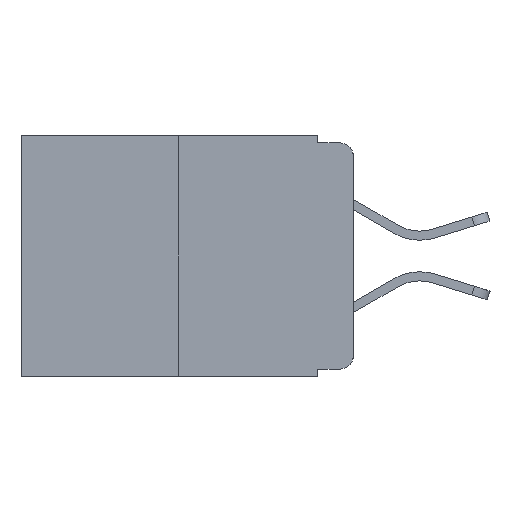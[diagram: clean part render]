
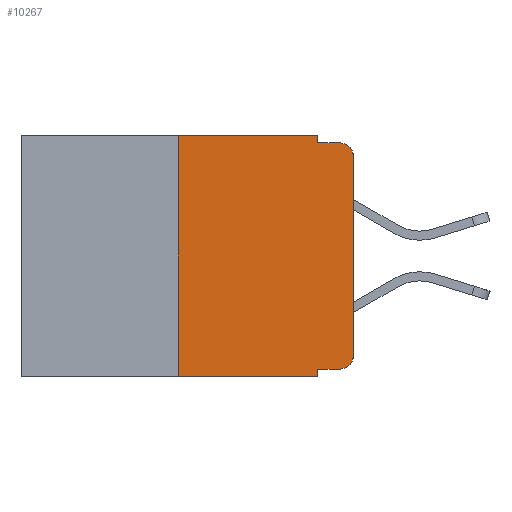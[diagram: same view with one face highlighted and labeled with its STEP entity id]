
A CAD part, left-side view. The second image highlights one B-rep face of the part: STEP entity #10267.
In plain terms, the highlighted planar face has unit normal (-1, 0, 0).
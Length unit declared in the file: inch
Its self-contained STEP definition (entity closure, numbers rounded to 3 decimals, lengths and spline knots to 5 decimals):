
#86 = CARTESIAN_POINT ( 'NONE',  ( 0., 0.051, -0.343 ) ) ;
#326 = CARTESIAN_POINT ( 'NONE',  ( 0., 0.02, -0.333 ) ) ;
#741 = CARTESIAN_POINT ( 'NONE',  ( 0., 0.02, -0.01 ) ) ;
#762 = DIRECTION ( 'NONE',  ( 0., 0., -1. ) ) ;
#869 = VERTEX_POINT ( 'NONE', #6838 ) ;
#930 = LINE ( 'NONE', #11428, #10359 ) ;
#1096 = DIRECTION ( 'NONE',  ( 0., -1., 0. ) ) ;
#1146 = DIRECTION ( 'NONE',  ( 0., 0., -1. ) ) ;
#1485 = EDGE_CURVE ( 'NONE', #869, #4838, #7308, .T. ) ;
#1521 = DIRECTION ( 'NONE',  ( 0., -1., 0. ) ) ;
#1691 = CARTESIAN_POINT ( 'NONE',  ( 0., 0.473, 0. ) ) ;
#1888 = ORIENTED_EDGE ( 'NONE', *, *, #10869, .T. ) ;
#2103 = ORIENTED_EDGE ( 'NONE', *, *, #10968, .F. ) ;
#2133 = ORIENTED_EDGE ( 'NONE', *, *, #5006, .T. ) ;
#2222 = CARTESIAN_POINT ( 'NONE',  ( 0., 0.051, -0.333 ) ) ;
#2382 = VECTOR ( 'NONE', #1096, 39.37008 ) ;
#2498 = CARTESIAN_POINT ( 'NONE',  ( 0., 0.051, -0.333 ) ) ;
#2697 = EDGE_CURVE ( 'NONE', #8519, #7471, #4111, .T. ) ;
#3133 = CARTESIAN_POINT ( 'NONE',  ( 0., 0.051, -0.01 ) ) ;
#3142 = LINE ( 'NONE', #2222, #10545 ) ;
#3174 = ORIENTED_EDGE ( 'NONE', *, *, #7615, .T. ) ;
#3338 = VERTEX_POINT ( 'NONE', #3133 ) ;
#3466 = CARTESIAN_POINT ( 'NONE',  ( 0., 0.051, -0.01 ) ) ;
#3538 = VERTEX_POINT ( 'NONE', #741 ) ;
#3566 = DIRECTION ( 'NONE',  ( 0., 0., -1. ) ) ;
#3585 = CARTESIAN_POINT ( 'NONE',  ( 0., 0., 0. ) ) ;
#3714 = LINE ( 'NONE', #3585, #6738 ) ;
#3739 = DIRECTION ( 'NONE',  ( -1., 0., 0. ) ) ;
#3763 = DIRECTION ( 'NONE',  ( 0., 0., 1. ) ) ;
#4007 = ORIENTED_EDGE ( 'NONE', *, *, #11514, .F. ) ;
#4111 = CIRCLE ( 'NONE', #6264, 0.02 ) ;
#4202 = LINE ( 'NONE', #6184, #2382 ) ;
#4651 = ORIENTED_EDGE ( 'NONE', *, *, #12097, .F. ) ;
#4686 = EDGE_CURVE ( 'NONE', #12040, #3338, #10063, .T. ) ;
#4838 = VERTEX_POINT ( 'NONE', #86 ) ;
#4857 = FACE_OUTER_BOUND ( 'NONE', #10212, .T. ) ;
#5006 = EDGE_CURVE ( 'NONE', #5683, #3538, #10392, .T. ) ;
#5345 = CARTESIAN_POINT ( 'NONE',  ( 0., 0., -0.03 ) ) ;
#5683 = VERTEX_POINT ( 'NONE', #5345 ) ;
#5799 = DIRECTION ( 'NONE',  ( 0., 0., -1. ) ) ;
#6101 = CARTESIAN_POINT ( 'NONE',  ( 0., 0.051, 0. ) ) ;
#6184 = CARTESIAN_POINT ( 'NONE',  ( 0., 0.473, 0. ) ) ;
#6264 = AXIS2_PLACEMENT_3D ( 'NONE', #6827, #3739, #5799 ) ;
#6509 = AXIS2_PLACEMENT_3D ( 'NONE', #12863, #7757, #8587 ) ;
#6738 = VECTOR ( 'NONE', #7641, 39.37008 ) ;
#6827 = CARTESIAN_POINT ( 'NONE',  ( 0., 0.02, -0.313 ) ) ;
#6838 = CARTESIAN_POINT ( 'NONE',  ( 0., 0.25, -0.343 ) ) ;
#6923 = CARTESIAN_POINT ( 'NONE',  ( 0., 0.25, 0. ) ) ;
#7249 = ORIENTED_EDGE ( 'NONE', *, *, #1485, .T. ) ;
#7257 = CARTESIAN_POINT ( 'NONE',  ( 0., 0.25, 0. ) ) ;
#7308 = LINE ( 'NONE', #8177, #12240 ) ;
#7348 = ORIENTED_EDGE ( 'NONE', *, *, #4686, .F. ) ;
#7381 = DIRECTION ( 'NONE',  ( 0., -1., 0. ) ) ;
#7471 = VERTEX_POINT ( 'NONE', #10618 ) ;
#7615 = EDGE_CURVE ( 'NONE', #7471, #5683, #3714, .T. ) ;
#7641 = DIRECTION ( 'NONE',  ( 0., 0., 1. ) ) ;
#7757 = DIRECTION ( 'NONE',  ( -1., 0., 0. ) ) ;
#7809 = AXIS2_PLACEMENT_3D ( 'NONE', #1691, #10832, #3566 ) ;
#8177 = CARTESIAN_POINT ( 'NONE',  ( 0., 0.473, -0.343 ) ) ;
#8360 = EDGE_CURVE ( 'NONE', #9010, #12040, #4202, .T. ) ;
#8445 = VERTEX_POINT ( 'NONE', #2498 ) ;
#8519 = VERTEX_POINT ( 'NONE', #326 ) ;
#8587 = DIRECTION ( 'NONE',  ( 0., 0., -1. ) ) ;
#8661 = LINE ( 'NONE', #3466, #11825 ) ;
#8771 = VECTOR ( 'NONE', #762, 39.37008 ) ;
#8960 = LINE ( 'NONE', #6923, #9270 ) ;
#9010 = VERTEX_POINT ( 'NONE', #7257 ) ;
#9270 = VECTOR ( 'NONE', #3763, 39.37008 ) ;
#10063 = LINE ( 'NONE', #10268, #8771 ) ;
#10212 = EDGE_LOOP ( 'NONE', ( #3174, #2133, #2103, #7348, #10924, #4007, #7249, #4651, #1888, #10511 ) ) ;
#10267 = ADVANCED_FACE ( 'NONE', ( #4857 ), #13105, .F. ) ;
#10268 = CARTESIAN_POINT ( 'NONE',  ( 0., 0.051, 0. ) ) ;
#10359 = VECTOR ( 'NONE', #1146, 39.37008 ) ;
#10392 = CIRCLE ( 'NONE', #6509, 0.02 ) ;
#10511 = ORIENTED_EDGE ( 'NONE', *, *, #2697, .T. ) ;
#10545 = VECTOR ( 'NONE', #7381, 39.37008 ) ;
#10618 = CARTESIAN_POINT ( 'NONE',  ( 0., 0., -0.313 ) ) ;
#10832 = DIRECTION ( 'NONE',  ( 1., 0., 0. ) ) ;
#10869 = EDGE_CURVE ( 'NONE', #8445, #8519, #3142, .T. ) ;
#10924 = ORIENTED_EDGE ( 'NONE', *, *, #8360, .F. ) ;
#10968 = EDGE_CURVE ( 'NONE', #3338, #3538, #8661, .T. ) ;
#11214 = DIRECTION ( 'NONE',  ( 0., -1., 0. ) ) ;
#11428 = CARTESIAN_POINT ( 'NONE',  ( 0., 0.051, 0. ) ) ;
#11514 = EDGE_CURVE ( 'NONE', #869, #9010, #8960, .T. ) ;
#11825 = VECTOR ( 'NONE', #1521, 39.37008 ) ;
#12040 = VERTEX_POINT ( 'NONE', #6101 ) ;
#12097 = EDGE_CURVE ( 'NONE', #8445, #4838, #930, .T. ) ;
#12240 = VECTOR ( 'NONE', #11214, 39.37008 ) ;
#12863 = CARTESIAN_POINT ( 'NONE',  ( 0., 0.02, -0.03 ) ) ;
#13105 = PLANE ( 'NONE',  #7809 ) ;
